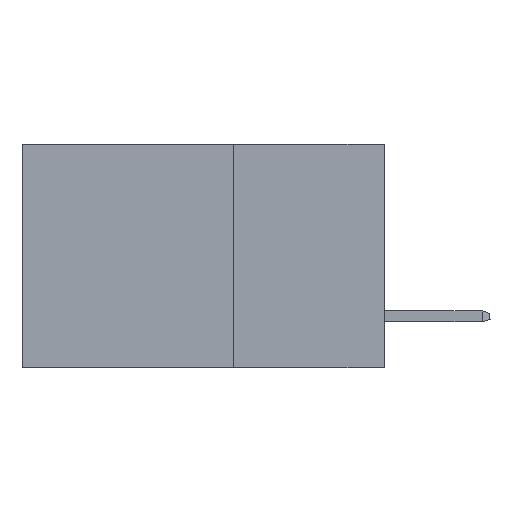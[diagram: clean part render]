
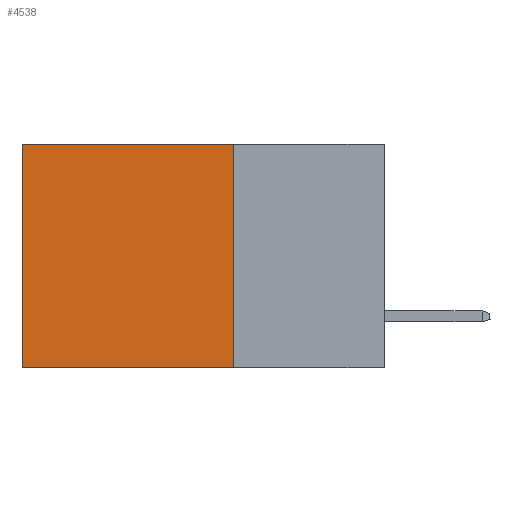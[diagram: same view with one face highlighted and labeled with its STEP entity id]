
A CAD part, left-side view. The second image highlights one B-rep face of the part: STEP entity #4538.
In plain terms, the highlighted planar face has unit normal (-1, 0, 0).
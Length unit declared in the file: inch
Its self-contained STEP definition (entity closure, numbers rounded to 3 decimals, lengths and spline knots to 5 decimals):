
#442 = VECTOR ( 'NONE', #24585, 39.37008 ) ;
#800 = VERTEX_POINT ( 'NONE', #1176 ) ;
#919 = CARTESIAN_POINT ( 'NONE',  ( 0.298, 0.25, 0. ) ) ;
#1176 = CARTESIAN_POINT ( 'NONE',  ( 0.298, 0.6, -0.37 ) ) ;
#1578 = EDGE_CURVE ( 'NONE', #10139, #12945, #19289, .T. ) ;
#4538 = ADVANCED_FACE ( 'NONE', ( #22466 ), #12934, .F. ) ;
#6224 = CARTESIAN_POINT ( 'NONE',  ( 0.298, 0.25, 0. ) ) ;
#7619 = CARTESIAN_POINT ( 'NONE',  ( 0.298, 0.6, 0. ) ) ;
#8507 = EDGE_LOOP ( 'NONE', ( #13990, #8638, #26271, #9942 ) ) ;
#8638 = ORIENTED_EDGE ( 'NONE', *, *, #24372, .F. ) ;
#9728 = CARTESIAN_POINT ( 'NONE',  ( 0.298, 0.25, 0. ) ) ;
#9942 = ORIENTED_EDGE ( 'NONE', *, *, #1578, .T. ) ;
#10139 = VERTEX_POINT ( 'NONE', #9728 ) ;
#10195 = LINE ( 'NONE', #11772, #14259 ) ;
#11299 = DIRECTION ( 'NONE',  ( 1., 0., 0. ) ) ;
#11772 = CARTESIAN_POINT ( 'NONE',  ( 0.298, 0.6, 0. ) ) ;
#12671 = AXIS2_PLACEMENT_3D ( 'NONE', #19752, #11299, #15307 ) ;
#12934 = PLANE ( 'NONE',  #12671 ) ;
#12945 = VERTEX_POINT ( 'NONE', #7619 ) ;
#13990 = ORIENTED_EDGE ( 'NONE', *, *, #14103, .T. ) ;
#14103 = EDGE_CURVE ( 'NONE', #12945, #800, #10195, .T. ) ;
#14259 = VECTOR ( 'NONE', #26857, 39.37008 ) ;
#14858 = LINE ( 'NONE', #6224, #442 ) ;
#15307 = DIRECTION ( 'NONE',  ( 0., 0., -1. ) ) ;
#15372 = CARTESIAN_POINT ( 'NONE',  ( 0.298, 0.25, -0.37 ) ) ;
#17776 = CARTESIAN_POINT ( 'NONE',  ( 0.298, 0.25, -0.37 ) ) ;
#18224 = LINE ( 'NONE', #15372, #18556 ) ;
#18556 = VECTOR ( 'NONE', #22180, 39.37008 ) ;
#19289 = LINE ( 'NONE', #919, #27112 ) ;
#19752 = CARTESIAN_POINT ( 'NONE',  ( 0.298, 0.25, 0. ) ) ;
#22180 = DIRECTION ( 'NONE',  ( 0., 1., 0. ) ) ;
#22466 = FACE_OUTER_BOUND ( 'NONE', #8507, .T. ) ;
#23976 = VERTEX_POINT ( 'NONE', #17776 ) ;
#24372 = EDGE_CURVE ( 'NONE', #23976, #800, #18224, .T. ) ;
#24585 = DIRECTION ( 'NONE',  ( 0., 0., -1. ) ) ;
#24653 = DIRECTION ( 'NONE',  ( 0., 1., 0. ) ) ;
#25561 = EDGE_CURVE ( 'NONE', #10139, #23976, #14858, .T. ) ;
#26271 = ORIENTED_EDGE ( 'NONE', *, *, #25561, .F. ) ;
#26857 = DIRECTION ( 'NONE',  ( 0., 0., -1. ) ) ;
#27112 = VECTOR ( 'NONE', #24653, 39.37008 ) ;
